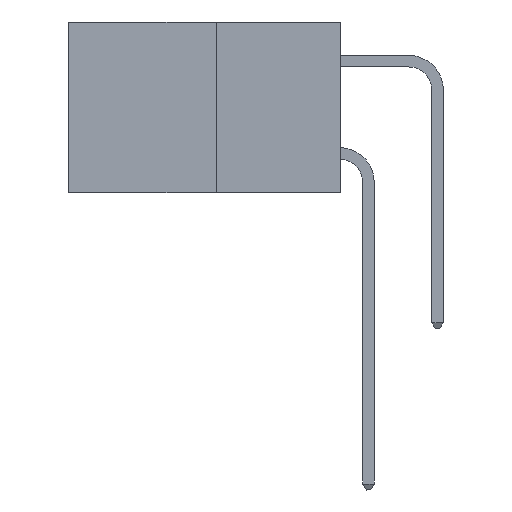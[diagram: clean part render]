
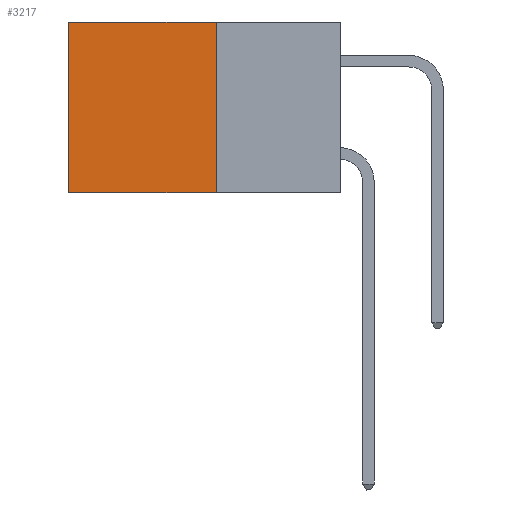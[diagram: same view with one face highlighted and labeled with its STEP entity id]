
A CAD part, left-side view. The second image highlights one B-rep face of the part: STEP entity #3217.
In plain terms, the highlighted planar face has unit normal (-1, 0, 0).
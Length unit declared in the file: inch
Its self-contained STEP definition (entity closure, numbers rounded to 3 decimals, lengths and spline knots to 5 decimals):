
#51 = FACE_OUTER_BOUND ( 'NONE', #6595, .T. ) ;
#200 = VECTOR ( 'NONE', #13107, 39.37008 ) ;
#2261 = ORIENTED_EDGE ( 'NONE', *, *, #3327, .F. ) ;
#2300 = CARTESIAN_POINT ( 'NONE',  ( 0.277, 0.27, -0.37 ) ) ;
#2461 = VECTOR ( 'NONE', #8862, 39.37008 ) ;
#2884 = VERTEX_POINT ( 'NONE', #2300 ) ;
#3217 = ADVANCED_FACE ( 'NONE', ( #51 ), #3609, .F. ) ;
#3327 = EDGE_CURVE ( 'NONE', #2884, #5403, #10654, .T. ) ;
#3609 = PLANE ( 'NONE',  #12059 ) ;
#4372 = EDGE_CURVE ( 'NONE', #6411, #2884, #9246, .T. ) ;
#5003 = ORIENTED_EDGE ( 'NONE', *, *, #13199, .T. ) ;
#5356 = ORIENTED_EDGE ( 'NONE', *, *, #4372, .F. ) ;
#5403 = VERTEX_POINT ( 'NONE', #12502 ) ;
#5540 = LINE ( 'NONE', #13218, #2461 ) ;
#5570 = CARTESIAN_POINT ( 'NONE',  ( 0.277, 0.27, 0. ) ) ;
#5575 = CARTESIAN_POINT ( 'NONE',  ( 0.277, 0.27, -0.37 ) ) ;
#5808 = DIRECTION ( 'NONE',  ( 0., 1., 0. ) ) ;
#6094 = DIRECTION ( 'NONE',  ( 1., 0., 0. ) ) ;
#6411 = VERTEX_POINT ( 'NONE', #5570 ) ;
#6595 = EDGE_LOOP ( 'NONE', ( #5003, #2261, #5356, #11128 ) ) ;
#7487 = DIRECTION ( 'NONE',  ( 0., 0., -1. ) ) ;
#7770 = VECTOR ( 'NONE', #5808, 39.37008 ) ;
#8862 = DIRECTION ( 'NONE',  ( 0., 0., -1. ) ) ;
#9246 = LINE ( 'NONE', #10856, #200 ) ;
#9632 = EDGE_CURVE ( 'NONE', #6411, #13622, #11068, .T. ) ;
#10130 = CARTESIAN_POINT ( 'NONE',  ( 0.277, 0.59, 0. ) ) ;
#10577 = CARTESIAN_POINT ( 'NONE',  ( 0.277, 0.27, -0.37 ) ) ;
#10654 = LINE ( 'NONE', #5575, #7770 ) ;
#10856 = CARTESIAN_POINT ( 'NONE',  ( 0.277, 0.27, -0.37 ) ) ;
#11068 = LINE ( 'NONE', #13959, #14243 ) ;
#11128 = ORIENTED_EDGE ( 'NONE', *, *, #9632, .T. ) ;
#12059 = AXIS2_PLACEMENT_3D ( 'NONE', #10577, #6094, #7487 ) ;
#12502 = CARTESIAN_POINT ( 'NONE',  ( 0.277, 0.59, -0.37 ) ) ;
#13107 = DIRECTION ( 'NONE',  ( 0., 0., -1. ) ) ;
#13199 = EDGE_CURVE ( 'NONE', #13622, #5403, #5540, .T. ) ;
#13218 = CARTESIAN_POINT ( 'NONE',  ( 0.277, 0.59, -0.37 ) ) ;
#13622 = VERTEX_POINT ( 'NONE', #10130 ) ;
#13939 = DIRECTION ( 'NONE',  ( 0., 1., 0. ) ) ;
#13959 = CARTESIAN_POINT ( 'NONE',  ( 0.277, 0.27, 0. ) ) ;
#14243 = VECTOR ( 'NONE', #13939, 39.37008 ) ;
